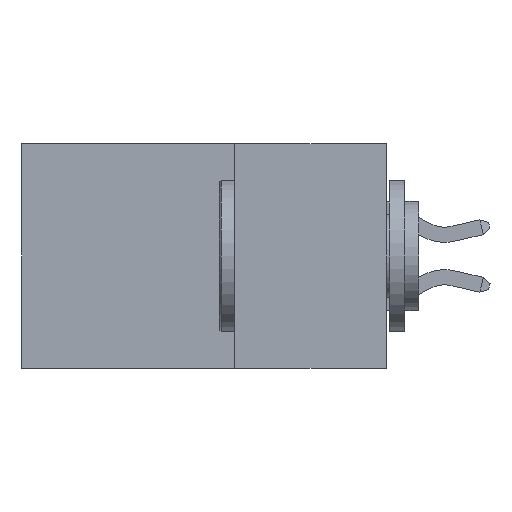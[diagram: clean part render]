
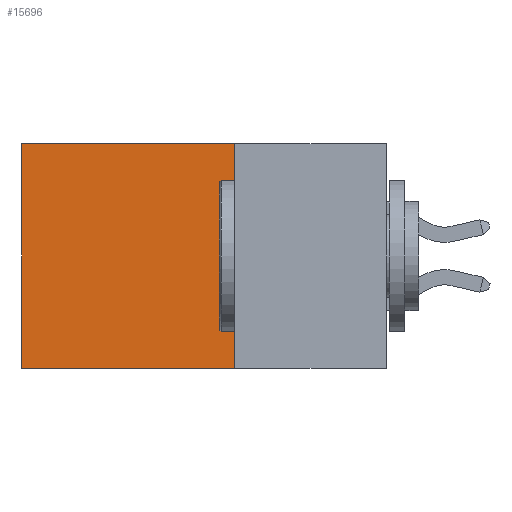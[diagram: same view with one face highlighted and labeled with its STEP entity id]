
A CAD part, left-side view. The second image highlights one B-rep face of the part: STEP entity #15696.
In plain terms, the highlighted planar face has unit normal (-1, 0, 0).
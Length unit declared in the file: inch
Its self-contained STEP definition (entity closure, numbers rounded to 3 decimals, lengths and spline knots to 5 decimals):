
#348 = DIRECTION ( 'NONE',  ( 0., 0., -1. ) ) ;
#500 = EDGE_CURVE ( 'NONE', #24929, #20208, #10069, .T. ) ;
#1264 = DIRECTION ( 'NONE',  ( 0., 1., 0. ) ) ;
#2522 = LINE ( 'NONE', #30245, #27147 ) ;
#3989 = VECTOR ( 'NONE', #7141, 39.37008 ) ;
#4463 = DIRECTION ( 'NONE',  ( 0., 0., -1. ) ) ;
#5721 = CARTESIAN_POINT ( 'NONE',  ( 0.298, 0.6, 0. ) ) ;
#6842 = AXIS2_PLACEMENT_3D ( 'NONE', #28273, #9127, #4463 ) ;
#7141 = DIRECTION ( 'NONE',  ( 0., 0., -1. ) ) ;
#7448 = CARTESIAN_POINT ( 'NONE',  ( 0.298, 0.25, 0. ) ) ;
#7465 = CARTESIAN_POINT ( 'NONE',  ( 0.298, 0.6, -0.37 ) ) ;
#8038 = LINE ( 'NONE', #7448, #3989 ) ;
#8892 = EDGE_CURVE ( 'NONE', #24929, #20428, #8038, .T. ) ;
#9127 = DIRECTION ( 'NONE',  ( 1., 0., 0. ) ) ;
#9479 = VECTOR ( 'NONE', #348, 39.37008 ) ;
#9594 = ORIENTED_EDGE ( 'NONE', *, *, #25320, .F. ) ;
#9840 = EDGE_CURVE ( 'NONE', #20208, #13851, #23678, .T. ) ;
#10069 = LINE ( 'NONE', #25122, #22761 ) ;
#10170 = ORIENTED_EDGE ( 'NONE', *, *, #9840, .T. ) ;
#12017 = CARTESIAN_POINT ( 'NONE',  ( 0.298, 0.6, 0. ) ) ;
#13851 = VERTEX_POINT ( 'NONE', #7465 ) ;
#15375 = FACE_OUTER_BOUND ( 'NONE', #25123, .T. ) ;
#15696 = ADVANCED_FACE ( 'NONE', ( #15375 ), #25955, .F. ) ;
#15949 = CARTESIAN_POINT ( 'NONE',  ( 0.298, 0.25, 0. ) ) ;
#16066 = ORIENTED_EDGE ( 'NONE', *, *, #8892, .F. ) ;
#18701 = CARTESIAN_POINT ( 'NONE',  ( 0.298, 0.25, -0.37 ) ) ;
#20208 = VERTEX_POINT ( 'NONE', #5721 ) ;
#20428 = VERTEX_POINT ( 'NONE', #18701 ) ;
#22761 = VECTOR ( 'NONE', #29966, 39.37008 ) ;
#23678 = LINE ( 'NONE', #12017, #9479 ) ;
#24929 = VERTEX_POINT ( 'NONE', #15949 ) ;
#25122 = CARTESIAN_POINT ( 'NONE',  ( 0.298, 0.25, 0. ) ) ;
#25123 = EDGE_LOOP ( 'NONE', ( #10170, #9594, #16066, #29491 ) ) ;
#25320 = EDGE_CURVE ( 'NONE', #20428, #13851, #2522, .T. ) ;
#25955 = PLANE ( 'NONE',  #6842 ) ;
#27147 = VECTOR ( 'NONE', #1264, 39.37008 ) ;
#28273 = CARTESIAN_POINT ( 'NONE',  ( 0.298, 0.25, 0. ) ) ;
#29491 = ORIENTED_EDGE ( 'NONE', *, *, #500, .T. ) ;
#29966 = DIRECTION ( 'NONE',  ( 0., 1., 0. ) ) ;
#30245 = CARTESIAN_POINT ( 'NONE',  ( 0.298, 0.25, -0.37 ) ) ;
